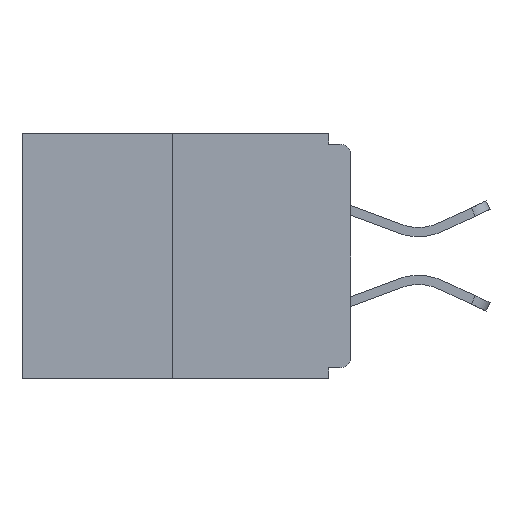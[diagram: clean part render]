
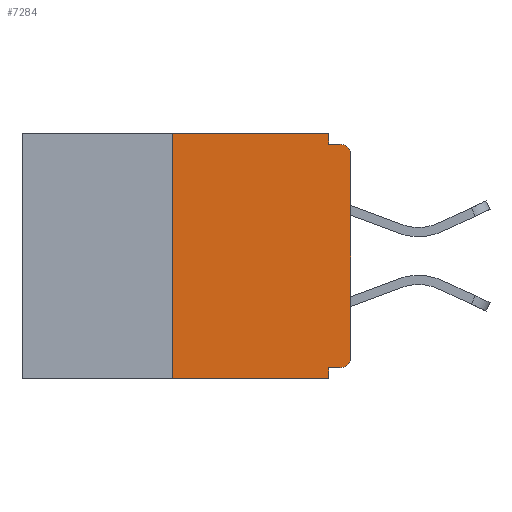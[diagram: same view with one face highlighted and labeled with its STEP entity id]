
A CAD part, left-side view. The second image highlights one B-rep face of the part: STEP entity #7284.
In plain terms, the highlighted planar face has unit normal (-1, 0, 0).
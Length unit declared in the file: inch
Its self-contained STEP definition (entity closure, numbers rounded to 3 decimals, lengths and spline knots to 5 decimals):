
#4 = CARTESIAN_POINT ( 'NONE',  ( 0., 0.25, 0. ) ) ;
#46 = VECTOR ( 'NONE', #5738, 39.37008 ) ;
#243 = LINE ( 'NONE', #3750, #10186 ) ;
#387 = CARTESIAN_POINT ( 'NONE',  ( 0., 0.46, 0. ) ) ;
#486 = DIRECTION ( 'NONE',  ( 0., 0., -1. ) ) ;
#773 = VERTEX_POINT ( 'NONE', #5936 ) ;
#1163 = ORIENTED_EDGE ( 'NONE', *, *, #9623, .F. ) ;
#1251 = ORIENTED_EDGE ( 'NONE', *, *, #11430, .T. ) ;
#1499 = LINE ( 'NONE', #387, #7063 ) ;
#1657 = EDGE_CURVE ( 'NONE', #3578, #3788, #2251, .T. ) ;
#1679 = LINE ( 'NONE', #9261, #10096 ) ;
#1868 = EDGE_CURVE ( 'NONE', #773, #2256, #3782, .T. ) ;
#1995 = CARTESIAN_POINT ( 'NONE',  ( 0., 0.031, -0.343 ) ) ;
#2045 = EDGE_CURVE ( 'NONE', #11421, #7597, #1499, .T. ) ;
#2070 = FACE_OUTER_BOUND ( 'NONE', #12373, .T. ) ;
#2251 = CIRCLE ( 'NONE', #3572, 0.015 ) ;
#2256 = VERTEX_POINT ( 'NONE', #7712 ) ;
#2329 = DIRECTION ( 'NONE',  ( 0., -1., 0. ) ) ;
#2789 = EDGE_CURVE ( 'NONE', #2256, #3578, #243, .T. ) ;
#2790 = VECTOR ( 'NONE', #9881, 39.37008 ) ;
#2819 = LINE ( 'NONE', #1995, #4785 ) ;
#3115 = ORIENTED_EDGE ( 'NONE', *, *, #2045, .F. ) ;
#3294 = ORIENTED_EDGE ( 'NONE', *, *, #4436, .F. ) ;
#3322 = VECTOR ( 'NONE', #9691, 39.37008 ) ;
#3325 = CARTESIAN_POINT ( 'NONE',  ( 0., 0.25, -0.343 ) ) ;
#3348 = CARTESIAN_POINT ( 'NONE',  ( 0., 0.031, 0. ) ) ;
#3572 = AXIS2_PLACEMENT_3D ( 'NONE', #5242, #9014, #486 ) ;
#3578 = VERTEX_POINT ( 'NONE', #8584 ) ;
#3750 = CARTESIAN_POINT ( 'NONE',  ( 0., 0., 0. ) ) ;
#3782 = CIRCLE ( 'NONE', #8892, 0.015 ) ;
#3788 = VERTEX_POINT ( 'NONE', #4168 ) ;
#3874 = DIRECTION ( 'NONE',  ( 0., 0., 1. ) ) ;
#4168 = CARTESIAN_POINT ( 'NONE',  ( 0., 0.015, -0.015 ) ) ;
#4280 = CARTESIAN_POINT ( 'NONE',  ( 0., 0.031, -0.328 ) ) ;
#4436 = EDGE_CURVE ( 'NONE', #9089, #3788, #1679, .T. ) ;
#4580 = AXIS2_PLACEMENT_3D ( 'NONE', #5750, #11459, #10531 ) ;
#4785 = VECTOR ( 'NONE', #8754, 39.37008 ) ;
#4942 = DIRECTION ( 'NONE',  ( -1., 0., 0. ) ) ;
#5242 = CARTESIAN_POINT ( 'NONE',  ( 0., 0.015, -0.03 ) ) ;
#5276 = LINE ( 'NONE', #7686, #3322 ) ;
#5293 = DIRECTION ( 'NONE',  ( 0., -1., 0. ) ) ;
#5738 = DIRECTION ( 'NONE',  ( 0., 0., 1. ) ) ;
#5750 = CARTESIAN_POINT ( 'NONE',  ( 0., 0.46, 0. ) ) ;
#5936 = CARTESIAN_POINT ( 'NONE',  ( 0., 0.015, -0.328 ) ) ;
#6021 = ORIENTED_EDGE ( 'NONE', *, *, #2789, .T. ) ;
#6436 = VERTEX_POINT ( 'NONE', #4280 ) ;
#6613 = CARTESIAN_POINT ( 'NONE',  ( 0., 0.031, -0.015 ) ) ;
#6655 = VERTEX_POINT ( 'NONE', #10726 ) ;
#6768 = PLANE ( 'NONE',  #4580 ) ;
#6775 = CARTESIAN_POINT ( 'NONE',  ( 0., 0.25, 0. ) ) ;
#6847 = CARTESIAN_POINT ( 'NONE',  ( 0., 0., -0.328 ) ) ;
#7063 = VECTOR ( 'NONE', #2329, 39.37008 ) ;
#7284 = ADVANCED_FACE ( 'NONE', ( #2070 ), #6768, .F. ) ;
#7410 = EDGE_CURVE ( 'NONE', #773, #6436, #11864, .T. ) ;
#7597 = VERTEX_POINT ( 'NONE', #10754 ) ;
#7649 = VECTOR ( 'NONE', #9733, 39.37008 ) ;
#7686 = CARTESIAN_POINT ( 'NONE',  ( 0., 0.46, -0.343 ) ) ;
#7712 = CARTESIAN_POINT ( 'NONE',  ( 0., 0., -0.313 ) ) ;
#7823 = ORIENTED_EDGE ( 'NONE', *, *, #1868, .T. ) ;
#7891 = ORIENTED_EDGE ( 'NONE', *, *, #8843, .F. ) ;
#8423 = EDGE_CURVE ( 'NONE', #6436, #6655, #2819, .T. ) ;
#8584 = CARTESIAN_POINT ( 'NONE',  ( 0., 0., -0.03 ) ) ;
#8754 = DIRECTION ( 'NONE',  ( 0., 0., -1. ) ) ;
#8843 = EDGE_CURVE ( 'NONE', #7597, #9089, #10143, .T. ) ;
#8892 = AXIS2_PLACEMENT_3D ( 'NONE', #9457, #4942, #9776 ) ;
#8947 = ORIENTED_EDGE ( 'NONE', *, *, #1657, .T. ) ;
#9014 = DIRECTION ( 'NONE',  ( -1., 0., 0. ) ) ;
#9089 = VERTEX_POINT ( 'NONE', #6613 ) ;
#9261 = CARTESIAN_POINT ( 'NONE',  ( 0., 0., -0.015 ) ) ;
#9457 = CARTESIAN_POINT ( 'NONE',  ( 0., 0.015, -0.313 ) ) ;
#9577 = VERTEX_POINT ( 'NONE', #3325 ) ;
#9623 = EDGE_CURVE ( 'NONE', #9577, #11421, #10432, .T. ) ;
#9691 = DIRECTION ( 'NONE',  ( 0., -1., 0. ) ) ;
#9733 = DIRECTION ( 'NONE',  ( 0., 1., 0. ) ) ;
#9776 = DIRECTION ( 'NONE',  ( 0., 0., -1. ) ) ;
#9881 = DIRECTION ( 'NONE',  ( 0., 0., -1. ) ) ;
#10096 = VECTOR ( 'NONE', #5293, 39.37008 ) ;
#10143 = LINE ( 'NONE', #3348, #2790 ) ;
#10186 = VECTOR ( 'NONE', #3874, 39.37008 ) ;
#10432 = LINE ( 'NONE', #4, #46 ) ;
#10531 = DIRECTION ( 'NONE',  ( 0., 0., -1. ) ) ;
#10726 = CARTESIAN_POINT ( 'NONE',  ( 0., 0.031, -0.343 ) ) ;
#10754 = CARTESIAN_POINT ( 'NONE',  ( 0., 0.031, 0. ) ) ;
#11421 = VERTEX_POINT ( 'NONE', #6775 ) ;
#11430 = EDGE_CURVE ( 'NONE', #9577, #6655, #5276, .T. ) ;
#11459 = DIRECTION ( 'NONE',  ( 1., 0., 0. ) ) ;
#11864 = LINE ( 'NONE', #6847, #7649 ) ;
#11961 = ORIENTED_EDGE ( 'NONE', *, *, #8423, .F. ) ;
#12373 = EDGE_LOOP ( 'NONE', ( #3115, #1163, #1251, #11961, #12425, #7823, #6021, #8947, #3294, #7891 ) ) ;
#12425 = ORIENTED_EDGE ( 'NONE', *, *, #7410, .F. ) ;
